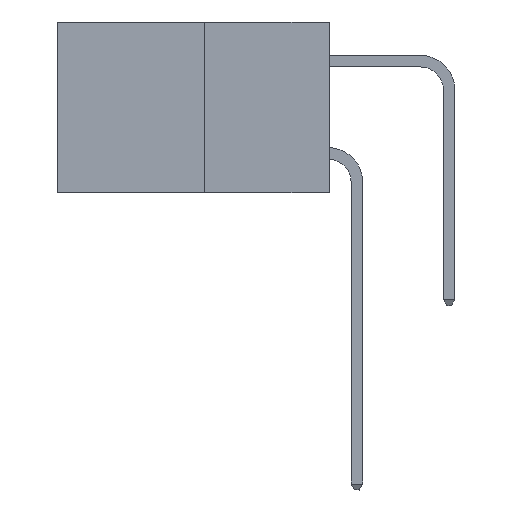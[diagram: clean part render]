
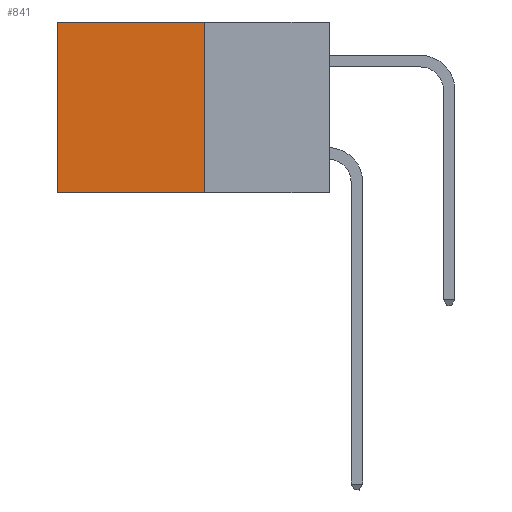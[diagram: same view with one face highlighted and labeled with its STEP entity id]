
A CAD part, left-side view. The second image highlights one B-rep face of the part: STEP entity #841.
In plain terms, the highlighted planar face has unit normal (-1, 0, 0).
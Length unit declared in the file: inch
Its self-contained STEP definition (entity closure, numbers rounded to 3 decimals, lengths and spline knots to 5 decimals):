
#21 = PLANE ( 'NONE',  #9201 ) ;
#841 = ADVANCED_FACE ( 'NONE', ( #30729 ), #21, .F. ) ;
#1359 = CARTESIAN_POINT ( 'NONE',  ( 0.277, 0.27, -0.37 ) ) ;
#3533 = ORIENTED_EDGE ( 'NONE', *, *, #7702, .T. ) ;
#4133 = CARTESIAN_POINT ( 'NONE',  ( 0.277, 0.27, -0.37 ) ) ;
#4713 = EDGE_CURVE ( 'NONE', #17002, #5912, #20479, .T. ) ;
#5912 = VERTEX_POINT ( 'NONE', #27779 ) ;
#7035 = DIRECTION ( 'NONE',  ( 0., 1., 0. ) ) ;
#7117 = EDGE_LOOP ( 'NONE', ( #28960, #18823, #28006, #3533 ) ) ;
#7702 = EDGE_CURVE ( 'NONE', #17002, #7778, #36622, .T. ) ;
#7778 = VERTEX_POINT ( 'NONE', #14443 ) ;
#9201 = AXIS2_PLACEMENT_3D ( 'NONE', #1359, #30071, #30031 ) ;
#10006 = CARTESIAN_POINT ( 'NONE',  ( 0.277, 0.59, -0.37 ) ) ;
#10321 = VECTOR ( 'NONE', #7035, 39.37008 ) ;
#11272 = CARTESIAN_POINT ( 'NONE',  ( 0.277, 0.27, -0.37 ) ) ;
#12803 = EDGE_CURVE ( 'NONE', #5912, #13507, #34992, .T. ) ;
#13129 = DIRECTION ( 'NONE',  ( 0., 0., -1. ) ) ;
#13507 = VERTEX_POINT ( 'NONE', #10006 ) ;
#13715 = VECTOR ( 'NONE', #34225, 39.37008 ) ;
#13933 = CARTESIAN_POINT ( 'NONE',  ( 0.277, 0.27, 0. ) ) ;
#14061 = DIRECTION ( 'NONE',  ( 0., 1., 0. ) ) ;
#14443 = CARTESIAN_POINT ( 'NONE',  ( 0.277, 0.59, 0. ) ) ;
#15915 = CARTESIAN_POINT ( 'NONE',  ( 0.277, 0.59, -0.37 ) ) ;
#16912 = EDGE_CURVE ( 'NONE', #7778, #13507, #27302, .T. ) ;
#17002 = VERTEX_POINT ( 'NONE', #32273 ) ;
#18823 = ORIENTED_EDGE ( 'NONE', *, *, #12803, .F. ) ;
#20479 = LINE ( 'NONE', #11272, #13715 ) ;
#26396 = VECTOR ( 'NONE', #13129, 39.37008 ) ;
#27302 = LINE ( 'NONE', #15915, #26396 ) ;
#27779 = CARTESIAN_POINT ( 'NONE',  ( 0.277, 0.27, -0.37 ) ) ;
#28006 = ORIENTED_EDGE ( 'NONE', *, *, #4713, .F. ) ;
#28960 = ORIENTED_EDGE ( 'NONE', *, *, #16912, .T. ) ;
#29121 = VECTOR ( 'NONE', #14061, 39.37008 ) ;
#30031 = DIRECTION ( 'NONE',  ( 0., 0., -1. ) ) ;
#30071 = DIRECTION ( 'NONE',  ( 1., 0., 0. ) ) ;
#30729 = FACE_OUTER_BOUND ( 'NONE', #7117, .T. ) ;
#32273 = CARTESIAN_POINT ( 'NONE',  ( 0.277, 0.27, 0. ) ) ;
#34225 = DIRECTION ( 'NONE',  ( 0., 0., -1. ) ) ;
#34992 = LINE ( 'NONE', #4133, #10321 ) ;
#36622 = LINE ( 'NONE', #13933, #29121 ) ;
